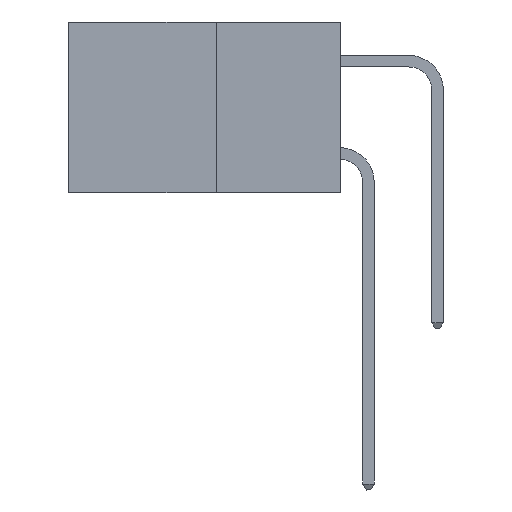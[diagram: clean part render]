
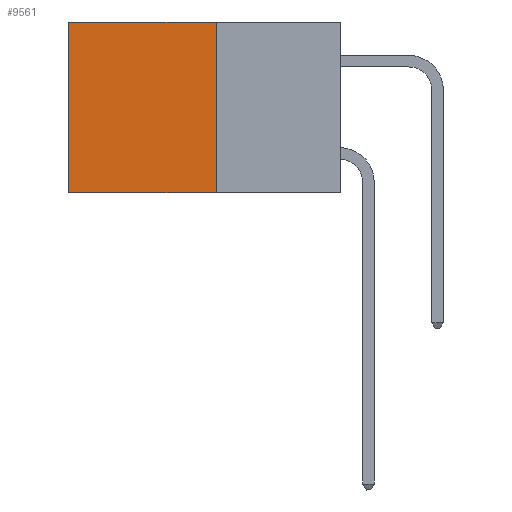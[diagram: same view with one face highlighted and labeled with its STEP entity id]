
A CAD part, left-side view. The second image highlights one B-rep face of the part: STEP entity #9561.
In plain terms, the highlighted planar face has unit normal (-1, 0, 0).
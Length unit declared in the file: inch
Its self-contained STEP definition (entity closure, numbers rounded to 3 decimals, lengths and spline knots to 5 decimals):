
#154 = CARTESIAN_POINT ( 'NONE',  ( 0.277, 0.59, 0. ) ) ;
#1395 = DIRECTION ( 'NONE',  ( 0., 0., -1. ) ) ;
#1696 = VECTOR ( 'NONE', #3274, 39.37008 ) ;
#2272 = VECTOR ( 'NONE', #6317, 39.37008 ) ;
#2790 = LINE ( 'NONE', #8683, #16319 ) ;
#3086 = PLANE ( 'NONE',  #6944 ) ;
#3274 = DIRECTION ( 'NONE',  ( 0., 0., -1. ) ) ;
#3424 = CARTESIAN_POINT ( 'NONE',  ( 0.277, 0.27, -0.37 ) ) ;
#4239 = EDGE_CURVE ( 'NONE', #11283, #10719, #15741, .T. ) ;
#4481 = DIRECTION ( 'NONE',  ( 1., 0., 0. ) ) ;
#4966 = CARTESIAN_POINT ( 'NONE',  ( 0.277, 0.27, -0.37 ) ) ;
#6317 = DIRECTION ( 'NONE',  ( 0., 1., 0. ) ) ;
#6944 = AXIS2_PLACEMENT_3D ( 'NONE', #12421, #4481, #13724 ) ;
#7277 = FACE_OUTER_BOUND ( 'NONE', #10235, .T. ) ;
#7547 = ORIENTED_EDGE ( 'NONE', *, *, #9640, .T. ) ;
#8683 = CARTESIAN_POINT ( 'NONE',  ( 0.277, 0.27, 0. ) ) ;
#8779 = CARTESIAN_POINT ( 'NONE',  ( 0.277, 0.59, -0.37 ) ) ;
#9561 = ADVANCED_FACE ( 'NONE', ( #7277 ), #3086, .F. ) ;
#9640 = EDGE_CURVE ( 'NONE', #11283, #14708, #2790, .T. ) ;
#9712 = LINE ( 'NONE', #10818, #13126 ) ;
#10235 = EDGE_LOOP ( 'NONE', ( #12840, #11326, #12819, #7547 ) ) ;
#10294 = CARTESIAN_POINT ( 'NONE',  ( 0.277, 0.27, -0.37 ) ) ;
#10719 = VERTEX_POINT ( 'NONE', #10294 ) ;
#10818 = CARTESIAN_POINT ( 'NONE',  ( 0.277, 0.59, -0.37 ) ) ;
#11283 = VERTEX_POINT ( 'NONE', #16508 ) ;
#11295 = DIRECTION ( 'NONE',  ( 0., 1., 0. ) ) ;
#11326 = ORIENTED_EDGE ( 'NONE', *, *, #16269, .F. ) ;
#11655 = EDGE_CURVE ( 'NONE', #14708, #13187, #9712, .T. ) ;
#12421 = CARTESIAN_POINT ( 'NONE',  ( 0.277, 0.27, -0.37 ) ) ;
#12819 = ORIENTED_EDGE ( 'NONE', *, *, #4239, .F. ) ;
#12840 = ORIENTED_EDGE ( 'NONE', *, *, #11655, .T. ) ;
#13126 = VECTOR ( 'NONE', #1395, 39.37008 ) ;
#13187 = VERTEX_POINT ( 'NONE', #8779 ) ;
#13724 = DIRECTION ( 'NONE',  ( 0., 0., -1. ) ) ;
#14708 = VERTEX_POINT ( 'NONE', #154 ) ;
#15741 = LINE ( 'NONE', #3424, #1696 ) ;
#16234 = LINE ( 'NONE', #4966, #2272 ) ;
#16269 = EDGE_CURVE ( 'NONE', #10719, #13187, #16234, .T. ) ;
#16319 = VECTOR ( 'NONE', #11295, 39.37008 ) ;
#16508 = CARTESIAN_POINT ( 'NONE',  ( 0.277, 0.27, 0. ) ) ;
